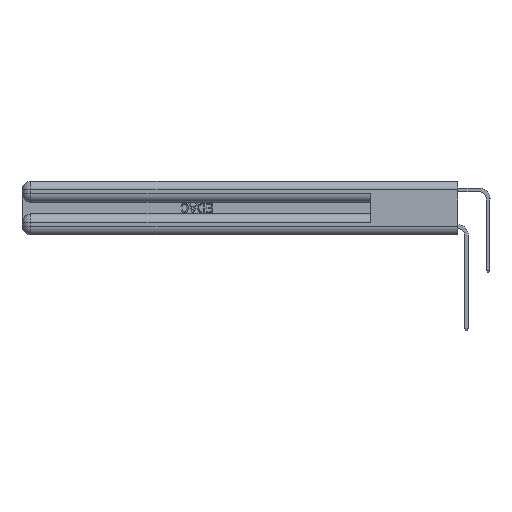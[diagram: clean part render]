
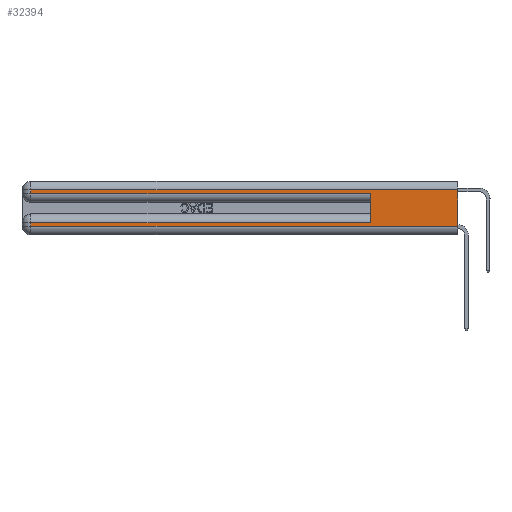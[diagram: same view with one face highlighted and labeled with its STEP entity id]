
A CAD part, left-side view. The second image highlights one B-rep face of the part: STEP entity #32394.
In plain terms, the highlighted planar face has unit normal (-1, 0, 0).
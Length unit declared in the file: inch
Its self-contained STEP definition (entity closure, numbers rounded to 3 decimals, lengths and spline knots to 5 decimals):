
#207 = EDGE_CURVE ( 'NONE', #10813, #33077, #15867, .T. ) ;
#260 = ORIENTED_EDGE ( 'NONE', *, *, #28107, .T. ) ;
#690 = ORIENTED_EDGE ( 'NONE', *, *, #27478, .F. ) ;
#1552 = VECTOR ( 'NONE', #4934, 39.37008 ) ;
#2005 = VECTOR ( 'NONE', #14973, 39.37008 ) ;
#2130 = CARTESIAN_POINT ( 'NONE',  ( 0., 0., 0.31 ) ) ;
#2315 = VECTOR ( 'NONE', #21291, 39.37008 ) ;
#3485 = ORIENTED_EDGE ( 'NONE', *, *, #20243, .T. ) ;
#4934 = DIRECTION ( 'NONE',  ( 0., 0., 1. ) ) ;
#5455 = CARTESIAN_POINT ( 'NONE',  ( 0., 0.6, 0.085 ) ) ;
#5677 = CARTESIAN_POINT ( 'NONE',  ( 0., 2.94, 0.37 ) ) ;
#6006 = EDGE_CURVE ( 'NONE', #30741, #30381, #28922, .T. ) ;
#6227 = EDGE_LOOP ( 'NONE', ( #690, #260, #34006, #29216, #8776, #7508, #8201, #3485 ) ) ;
#6639 = VERTEX_POINT ( 'NONE', #16487 ) ;
#7508 = ORIENTED_EDGE ( 'NONE', *, *, #28115, .T. ) ;
#8201 = ORIENTED_EDGE ( 'NONE', *, *, #207, .T. ) ;
#8491 = VECTOR ( 'NONE', #19017, 39.37008 ) ;
#8776 = ORIENTED_EDGE ( 'NONE', *, *, #6006, .F. ) ;
#8848 = EDGE_CURVE ( 'NONE', #6639, #11140, #35065, .T. ) ;
#8860 = LINE ( 'NONE', #32458, #13172 ) ;
#10076 = CARTESIAN_POINT ( 'NONE',  ( 0., 0.6, 0.145 ) ) ;
#10256 = CARTESIAN_POINT ( 'NONE',  ( 0., 2.94, 0.085 ) ) ;
#10711 = VECTOR ( 'NONE', #30670, 39.37008 ) ;
#10813 = VERTEX_POINT ( 'NONE', #10256 ) ;
#11140 = VERTEX_POINT ( 'NONE', #18245 ) ;
#13172 = VECTOR ( 'NONE', #18359, 39.37008 ) ;
#13781 = CARTESIAN_POINT ( 'NONE',  ( 0., 2.94, 0.06 ) ) ;
#14095 = FACE_OUTER_BOUND ( 'NONE', #6227, .T. ) ;
#14317 = LINE ( 'NONE', #35529, #18684 ) ;
#14836 = CARTESIAN_POINT ( 'NONE',  ( 0., 2.94, 0.37 ) ) ;
#14973 = DIRECTION ( 'NONE',  ( 0., 0., -1. ) ) ;
#15336 = LINE ( 'NONE', #2130, #2315 ) ;
#15867 = LINE ( 'NONE', #5677, #10711 ) ;
#16487 = CARTESIAN_POINT ( 'NONE',  ( 0., 2.94, 0.31 ) ) ;
#18245 = CARTESIAN_POINT ( 'NONE',  ( 0., 2.94, 0.285 ) ) ;
#18359 = DIRECTION ( 'NONE',  ( 0., 1., 0. ) ) ;
#18586 = VERTEX_POINT ( 'NONE', #23603 ) ;
#18684 = VECTOR ( 'NONE', #30206, 39.37008 ) ;
#19017 = DIRECTION ( 'NONE',  ( 0., -1., 0. ) ) ;
#20243 = EDGE_CURVE ( 'NONE', #33077, #18586, #27547, .T. ) ;
#20497 = CARTESIAN_POINT ( 'NONE',  ( 0., 0.6, 0.285 ) ) ;
#20764 = CARTESIAN_POINT ( 'NONE',  ( 0., 0., 0.06 ) ) ;
#20945 = VERTEX_POINT ( 'NONE', #26788 ) ;
#21291 = DIRECTION ( 'NONE',  ( 0., 1., 0. ) ) ;
#21619 = DIRECTION ( 'NONE',  ( 1., 0., 0. ) ) ;
#22773 = VECTOR ( 'NONE', #25889, 39.37008 ) ;
#23255 = LINE ( 'NONE', #27173, #8491 ) ;
#23603 = CARTESIAN_POINT ( 'NONE',  ( 0., 0., 0.06 ) ) ;
#25889 = DIRECTION ( 'NONE',  ( 0., -1., 0. ) ) ;
#26788 = CARTESIAN_POINT ( 'NONE',  ( 0., 0., 0.31 ) ) ;
#27075 = CARTESIAN_POINT ( 'NONE',  ( 0., 0., 0.37 ) ) ;
#27173 = CARTESIAN_POINT ( 'NONE',  ( 0., 0., 0.285 ) ) ;
#27478 = EDGE_CURVE ( 'NONE', #20945, #18586, #14317, .T. ) ;
#27547 = LINE ( 'NONE', #20764, #22773 ) ;
#28107 = EDGE_CURVE ( 'NONE', #20945, #6639, #15336, .T. ) ;
#28115 = EDGE_CURVE ( 'NONE', #30741, #10813, #8860, .T. ) ;
#28922 = LINE ( 'NONE', #10076, #1552 ) ;
#29216 = ORIENTED_EDGE ( 'NONE', *, *, #35035, .T. ) ;
#30206 = DIRECTION ( 'NONE',  ( 0., 0., -1. ) ) ;
#30381 = VERTEX_POINT ( 'NONE', #20497 ) ;
#30670 = DIRECTION ( 'NONE',  ( 0., 0., -1. ) ) ;
#30741 = VERTEX_POINT ( 'NONE', #5455 ) ;
#32394 = ADVANCED_FACE ( 'NONE', ( #14095 ), #32792, .F. ) ;
#32458 = CARTESIAN_POINT ( 'NONE',  ( 0., 0., 0.085 ) ) ;
#32792 = PLANE ( 'NONE',  #34445 ) ;
#33077 = VERTEX_POINT ( 'NONE', #13781 ) ;
#34006 = ORIENTED_EDGE ( 'NONE', *, *, #8848, .T. ) ;
#34445 = AXIS2_PLACEMENT_3D ( 'NONE', #27075, #21619, #35579 ) ;
#35035 = EDGE_CURVE ( 'NONE', #11140, #30381, #23255, .T. ) ;
#35065 = LINE ( 'NONE', #14836, #2005 ) ;
#35529 = CARTESIAN_POINT ( 'NONE',  ( 0., 0., 0.37 ) ) ;
#35579 = DIRECTION ( 'NONE',  ( 0., 0., -1. ) ) ;
